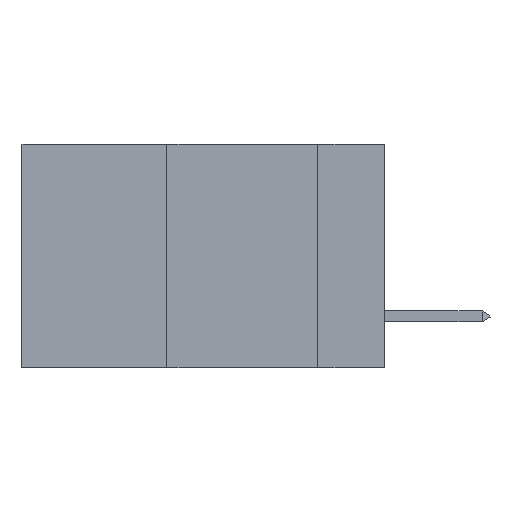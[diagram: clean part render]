
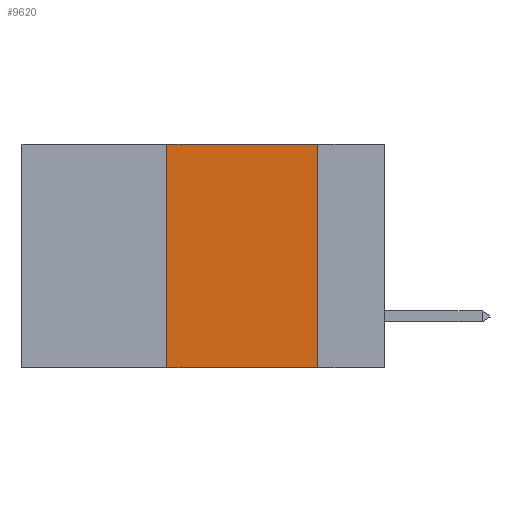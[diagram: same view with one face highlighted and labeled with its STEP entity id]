
A CAD part, left-side view. The second image highlights one B-rep face of the part: STEP entity #9620.
In plain terms, the highlighted planar face has unit normal (-1, 0, 0).
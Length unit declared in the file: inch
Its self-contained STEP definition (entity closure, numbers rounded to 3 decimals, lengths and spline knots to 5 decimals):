
#181 = EDGE_CURVE ( 'NONE', #13189, #397, #10371, .T. ) ;
#397 = VERTEX_POINT ( 'NONE', #10666 ) ;
#1848 = VECTOR ( 'NONE', #4319, 39.37008 ) ;
#1908 = VERTEX_POINT ( 'NONE', #7050 ) ;
#3123 = ORIENTED_EDGE ( 'NONE', *, *, #10337, .F. ) ;
#3336 = EDGE_CURVE ( 'NONE', #1908, #10318, #10879, .T. ) ;
#3599 = FACE_OUTER_BOUND ( 'NONE', #5260, .T. ) ;
#3849 = LINE ( 'NONE', #4396, #1848 ) ;
#4319 = DIRECTION ( 'NONE',  ( 0., 0., -1. ) ) ;
#4396 = CARTESIAN_POINT ( 'NONE',  ( 0., 0.11, 0. ) ) ;
#4467 = AXIS2_PLACEMENT_3D ( 'NONE', #21933, #23775, #7475 ) ;
#5260 = EDGE_LOOP ( 'NONE', ( #3123, #18659, #6422, #8750 ) ) ;
#5800 = PLANE ( 'NONE',  #4467 ) ;
#6422 = ORIENTED_EDGE ( 'NONE', *, *, #20219, .F. ) ;
#7050 = CARTESIAN_POINT ( 'NONE',  ( 0., 0.36, -0.37 ) ) ;
#7134 = VECTOR ( 'NONE', #14084, 39.37008 ) ;
#7475 = DIRECTION ( 'NONE',  ( 0., 0., -1. ) ) ;
#8750 = ORIENTED_EDGE ( 'NONE', *, *, #3336, .T. ) ;
#9620 = ADVANCED_FACE ( 'NONE', ( #3599 ), #5800, .F. ) ;
#10318 = VERTEX_POINT ( 'NONE', #15464 ) ;
#10337 = EDGE_CURVE ( 'NONE', #397, #10318, #3849, .T. ) ;
#10371 = LINE ( 'NONE', #14797, #23022 ) ;
#10666 = CARTESIAN_POINT ( 'NONE',  ( 0., 0.11, 0. ) ) ;
#10879 = LINE ( 'NONE', #14005, #7134 ) ;
#13189 = VERTEX_POINT ( 'NONE', #13764 ) ;
#13764 = CARTESIAN_POINT ( 'NONE',  ( 0., 0.36, 0. ) ) ;
#14005 = CARTESIAN_POINT ( 'NONE',  ( 0., 0.6, -0.37 ) ) ;
#14084 = DIRECTION ( 'NONE',  ( 0., -1., 0. ) ) ;
#14245 = VECTOR ( 'NONE', #21773, 39.37008 ) ;
#14797 = CARTESIAN_POINT ( 'NONE',  ( 0., 0.6, 0. ) ) ;
#15464 = CARTESIAN_POINT ( 'NONE',  ( 0., 0.11, -0.37 ) ) ;
#18163 = CARTESIAN_POINT ( 'NONE',  ( 0., 0.36, 0. ) ) ;
#18659 = ORIENTED_EDGE ( 'NONE', *, *, #181, .F. ) ;
#19161 = LINE ( 'NONE', #18163, #14245 ) ;
#20216 = DIRECTION ( 'NONE',  ( 0., -1., 0. ) ) ;
#20219 = EDGE_CURVE ( 'NONE', #1908, #13189, #19161, .T. ) ;
#21773 = DIRECTION ( 'NONE',  ( 0., 0., 1. ) ) ;
#21933 = CARTESIAN_POINT ( 'NONE',  ( 0., 0.6, 0. ) ) ;
#23022 = VECTOR ( 'NONE', #20216, 39.37008 ) ;
#23775 = DIRECTION ( 'NONE',  ( 1., 0., 0. ) ) ;
